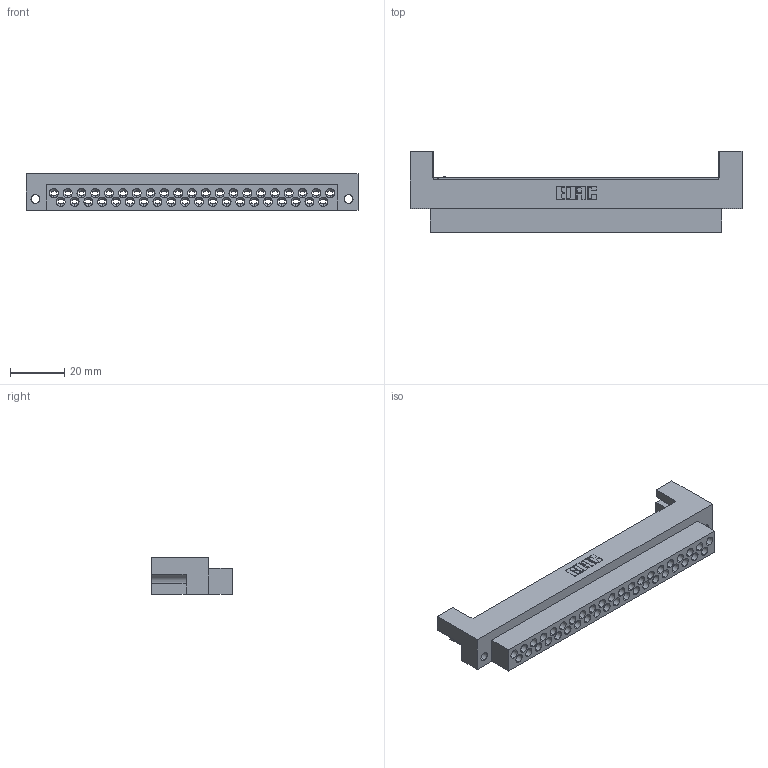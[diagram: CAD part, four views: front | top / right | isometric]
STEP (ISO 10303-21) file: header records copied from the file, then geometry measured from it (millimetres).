
FILE_DESCRIPTION (( 'STEP AP203' ), '1' );
FILE_NAME ('415-041-000-212.STEP', '2020-03-12T19:44:45', ( '' ), ( '' ), 'SwSTEP 2.0', 'SolidWorks 2016', '' );
FILE_SCHEMA (( 'CONFIG_CONTROL_DESIGN' ));
Length unit declared in the file: millimetre
Products named in the file (2): 415-041-000-212; 415-210-001_415-210-041-212
Assembly tree (1 placements, depth 2):
  415-041-000-212
    415-210-001_415-210-041-212
Bounding box: 122.07 x 29.77 x 13.49 mm (x, y, z)
Volume: 20154.4 mm3; surface area: 19772.3 mm2
Topology: 1 solids, 1 shells, 1226 faces, 3644 edges, 2387 vertices
Faces by surface type: plane 953, cylinder 128, cone 123, bspline 22
Entity records: 42369 total; most frequent: CARTESIAN_POINT 9823, ORIENTED_EDGE 7288, DIRECTION 6069, EDGE_CURVE 3644, VECTOR 2563, LINE 2563, VERTEX_POINT 2387, AXIS2_PLACEMENT_3D 1753
